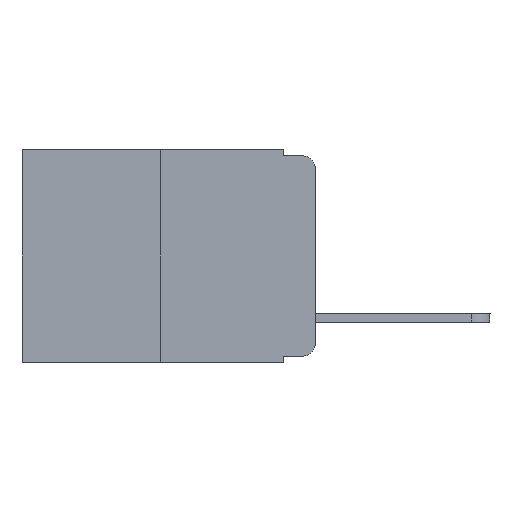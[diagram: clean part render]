
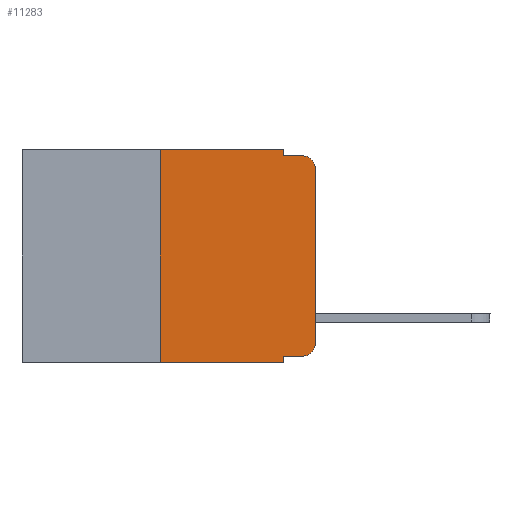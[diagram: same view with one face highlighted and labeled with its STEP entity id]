
A CAD part, left-side view. The second image highlights one B-rep face of the part: STEP entity #11283.
In plain terms, the highlighted planar face has unit normal (-1, 0, 0).
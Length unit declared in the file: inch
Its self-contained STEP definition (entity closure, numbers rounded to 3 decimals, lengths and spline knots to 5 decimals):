
#54 = VECTOR ( 'NONE', #9226, 39.37008 ) ;
#79 = CARTESIAN_POINT ( 'NONE',  ( 0., 0.051, -0.343 ) ) ;
#87 = LINE ( 'NONE', #140, #11435 ) ;
#140 = CARTESIAN_POINT ( 'NONE',  ( 0., 0.051, 0. ) ) ;
#203 = AXIS2_PLACEMENT_3D ( 'NONE', #8186, #2718, #855 ) ;
#744 = DIRECTION ( 'NONE',  ( -1., 0., 0. ) ) ;
#798 = CARTESIAN_POINT ( 'NONE',  ( 0., 0.051, -0.333 ) ) ;
#855 = DIRECTION ( 'NONE',  ( 0., 0., -1. ) ) ;
#908 = DIRECTION ( 'NONE',  ( 0., 0., -1. ) ) ;
#1181 = CARTESIAN_POINT ( 'NONE',  ( 0., 0.25, 0. ) ) ;
#1289 = ORIENTED_EDGE ( 'NONE', *, *, #9156, .F. ) ;
#1349 = EDGE_CURVE ( 'NONE', #7656, #1356, #6625, .T. ) ;
#1356 = VERTEX_POINT ( 'NONE', #9613 ) ;
#1403 = PLANE ( 'NONE',  #6693 ) ;
#1547 = EDGE_CURVE ( 'NONE', #2472, #5646, #7266, .T. ) ;
#1610 = DIRECTION ( 'NONE',  ( 0., -1., 0. ) ) ;
#1636 = DIRECTION ( 'NONE',  ( 0., 0., 1. ) ) ;
#1648 = CARTESIAN_POINT ( 'NONE',  ( 0., 0.25, -0.343 ) ) ;
#1880 = EDGE_CURVE ( 'NONE', #9843, #7656, #7919, .T. ) ;
#1923 = DIRECTION ( 'NONE',  ( 0., -1., 0. ) ) ;
#1946 = VECTOR ( 'NONE', #1610, 39.37008 ) ;
#1995 = CARTESIAN_POINT ( 'NONE',  ( 0., 0., -0.313 ) ) ;
#2221 = VERTEX_POINT ( 'NONE', #7590 ) ;
#2472 = VERTEX_POINT ( 'NONE', #1648 ) ;
#2477 = DIRECTION ( 'NONE',  ( 0., -1., 0. ) ) ;
#2637 = VERTEX_POINT ( 'NONE', #1995 ) ;
#2718 = DIRECTION ( 'NONE',  ( -1., 0., 0. ) ) ;
#2732 = VERTEX_POINT ( 'NONE', #11473 ) ;
#2859 = LINE ( 'NONE', #1181, #54 ) ;
#2872 = CARTESIAN_POINT ( 'NONE',  ( 0., 0.02, -0.333 ) ) ;
#2907 = EDGE_CURVE ( 'NONE', #8701, #1356, #5501, .T. ) ;
#3064 = CARTESIAN_POINT ( 'NONE',  ( 0., 0.051, -0.01 ) ) ;
#3127 = CARTESIAN_POINT ( 'NONE',  ( 0., 0.473, 0. ) ) ;
#3260 = DIRECTION ( 'NONE',  ( 1., 0., 0. ) ) ;
#3595 = VECTOR ( 'NONE', #9466, 39.37008 ) ;
#3606 = LINE ( 'NONE', #798, #7330 ) ;
#3827 = EDGE_CURVE ( 'NONE', #2637, #8701, #10635, .T. ) ;
#3860 = EDGE_CURVE ( 'NONE', #2732, #9111, #3606, .T. ) ;
#4154 = DIRECTION ( 'NONE',  ( 0., 0., -1. ) ) ;
#4174 = ORIENTED_EDGE ( 'NONE', *, *, #11151, .F. ) ;
#4268 = ORIENTED_EDGE ( 'NONE', *, *, #2907, .T. ) ;
#4282 = FACE_OUTER_BOUND ( 'NONE', #9993, .T. ) ;
#4892 = VECTOR ( 'NONE', #2477, 39.37008 ) ;
#5224 = CARTESIAN_POINT ( 'NONE',  ( 0., 0., 0. ) ) ;
#5301 = LINE ( 'NONE', #7129, #1946 ) ;
#5501 = CIRCLE ( 'NONE', #8533, 0.02 ) ;
#5646 = VERTEX_POINT ( 'NONE', #79 ) ;
#5821 = CARTESIAN_POINT ( 'NONE',  ( 0., 0.051, 0. ) ) ;
#5838 = CARTESIAN_POINT ( 'NONE',  ( 0., 0.051, -0.01 ) ) ;
#6123 = CARTESIAN_POINT ( 'NONE',  ( 0., 0.051, 0. ) ) ;
#6375 = VECTOR ( 'NONE', #1636, 39.37008 ) ;
#6625 = LINE ( 'NONE', #3064, #9268 ) ;
#6693 = AXIS2_PLACEMENT_3D ( 'NONE', #3127, #3260, #4154 ) ;
#7129 = CARTESIAN_POINT ( 'NONE',  ( 0., 0.473, 0. ) ) ;
#7266 = LINE ( 'NONE', #10058, #4892 ) ;
#7330 = VECTOR ( 'NONE', #1923, 39.37008 ) ;
#7349 = EDGE_CURVE ( 'NONE', #9111, #2637, #8555, .T. ) ;
#7383 = DIRECTION ( 'NONE',  ( 0., 0., -1. ) ) ;
#7555 = ORIENTED_EDGE ( 'NONE', *, *, #7349, .T. ) ;
#7574 = DIRECTION ( 'NONE',  ( 0., -1., 0. ) ) ;
#7590 = CARTESIAN_POINT ( 'NONE',  ( 0., 0.25, 0. ) ) ;
#7656 = VERTEX_POINT ( 'NONE', #5838 ) ;
#7919 = LINE ( 'NONE', #5821, #3595 ) ;
#8186 = CARTESIAN_POINT ( 'NONE',  ( 0., 0.02, -0.313 ) ) ;
#8533 = AXIS2_PLACEMENT_3D ( 'NONE', #8900, #744, #908 ) ;
#8555 = CIRCLE ( 'NONE', #203, 0.02 ) ;
#8685 = ORIENTED_EDGE ( 'NONE', *, *, #1880, .F. ) ;
#8701 = VERTEX_POINT ( 'NONE', #9312 ) ;
#8900 = CARTESIAN_POINT ( 'NONE',  ( 0., 0.02, -0.03 ) ) ;
#9017 = ORIENTED_EDGE ( 'NONE', *, *, #3827, .T. ) ;
#9111 = VERTEX_POINT ( 'NONE', #2872 ) ;
#9156 = EDGE_CURVE ( 'NONE', #2732, #5646, #87, .T. ) ;
#9226 = DIRECTION ( 'NONE',  ( 0., 0., 1. ) ) ;
#9268 = VECTOR ( 'NONE', #7574, 39.37008 ) ;
#9310 = ORIENTED_EDGE ( 'NONE', *, *, #1349, .F. ) ;
#9312 = CARTESIAN_POINT ( 'NONE',  ( 0., 0., -0.03 ) ) ;
#9466 = DIRECTION ( 'NONE',  ( 0., 0., -1. ) ) ;
#9613 = CARTESIAN_POINT ( 'NONE',  ( 0., 0.02, -0.01 ) ) ;
#9843 = VERTEX_POINT ( 'NONE', #6123 ) ;
#9980 = ORIENTED_EDGE ( 'NONE', *, *, #1547, .T. ) ;
#9993 = EDGE_LOOP ( 'NONE', ( #9017, #4268, #9310, #8685, #4174, #10404, #9980, #1289, #11184, #7555 ) ) ;
#10058 = CARTESIAN_POINT ( 'NONE',  ( 0., 0.473, -0.343 ) ) ;
#10404 = ORIENTED_EDGE ( 'NONE', *, *, #10846, .F. ) ;
#10635 = LINE ( 'NONE', #5224, #6375 ) ;
#10846 = EDGE_CURVE ( 'NONE', #2472, #2221, #2859, .T. ) ;
#11151 = EDGE_CURVE ( 'NONE', #2221, #9843, #5301, .T. ) ;
#11184 = ORIENTED_EDGE ( 'NONE', *, *, #3860, .T. ) ;
#11283 = ADVANCED_FACE ( 'NONE', ( #4282 ), #1403, .F. ) ;
#11435 = VECTOR ( 'NONE', #7383, 39.37008 ) ;
#11473 = CARTESIAN_POINT ( 'NONE',  ( 0., 0.051, -0.333 ) ) ;
